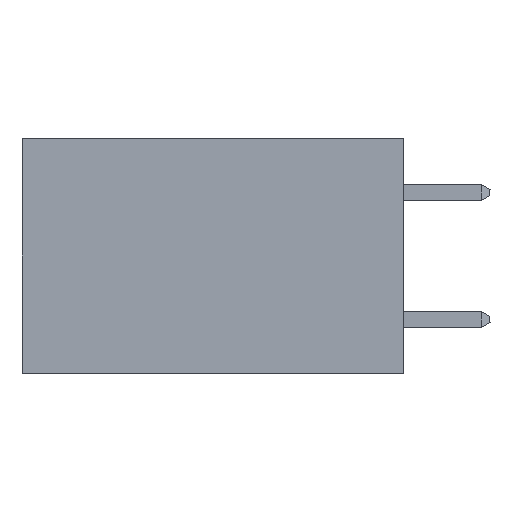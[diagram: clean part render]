
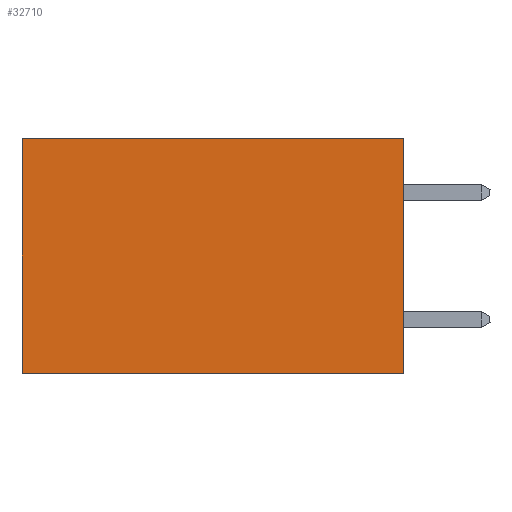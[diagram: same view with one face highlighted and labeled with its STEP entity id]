
A CAD part, left-side view. The second image highlights one B-rep face of the part: STEP entity #32710.
In plain terms, the highlighted planar face has unit normal (-1, 0, 0).
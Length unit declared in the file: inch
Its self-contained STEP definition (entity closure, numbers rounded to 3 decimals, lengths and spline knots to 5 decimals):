
#2787 = ORIENTED_EDGE ( 'NONE', *, *, #8721, .T. ) ;
#2903 = VERTEX_POINT ( 'NONE', #18863 ) ;
#3817 = ORIENTED_EDGE ( 'NONE', *, *, #26472, .T. ) ;
#4316 = CARTESIAN_POINT ( 'NONE',  ( 0.2875, 0.6, -0.37 ) ) ;
#5129 = DIRECTION ( 'NONE',  ( 1., 0., 0. ) ) ;
#7043 = DIRECTION ( 'NONE',  ( 0., 1., 0. ) ) ;
#7102 = CARTESIAN_POINT ( 'NONE',  ( 0.2875, 0., 0. ) ) ;
#7172 = LINE ( 'NONE', #17363, #12682 ) ;
#8721 = EDGE_CURVE ( 'NONE', #2903, #32211, #14900, .T. ) ;
#10259 = DIRECTION ( 'NONE',  ( 0., 0., -1. ) ) ;
#10766 = EDGE_LOOP ( 'NONE', ( #3817, #18517, #32597, #2787 ) ) ;
#11754 = CARTESIAN_POINT ( 'NONE',  ( 0.2875, 0.6, 0. ) ) ;
#12483 = EDGE_CURVE ( 'NONE', #2903, #37569, #7172, .T. ) ;
#12682 = VECTOR ( 'NONE', #14166, 39.37008 ) ;
#14070 = DIRECTION ( 'NONE',  ( 0., 0., -1. ) ) ;
#14166 = DIRECTION ( 'NONE',  ( 0., 0., -1. ) ) ;
#14900 = LINE ( 'NONE', #7102, #30327 ) ;
#16572 = DIRECTION ( 'NONE',  ( 0., 1., 0. ) ) ;
#17088 = VECTOR ( 'NONE', #7043, 39.37008 ) ;
#17363 = CARTESIAN_POINT ( 'NONE',  ( 0.2875, 0., 0. ) ) ;
#18517 = ORIENTED_EDGE ( 'NONE', *, *, #37823, .F. ) ;
#18863 = CARTESIAN_POINT ( 'NONE',  ( 0.2875, 0., 0. ) ) ;
#20298 = VERTEX_POINT ( 'NONE', #4316 ) ;
#20973 = PLANE ( 'NONE',  #25072 ) ;
#24264 = VECTOR ( 'NONE', #10259, 39.37008 ) ;
#24602 = LINE ( 'NONE', #32791, #17088 ) ;
#25072 = AXIS2_PLACEMENT_3D ( 'NONE', #26981, #5129, #14070 ) ;
#26472 = EDGE_CURVE ( 'NONE', #32211, #20298, #32759, .T. ) ;
#26981 = CARTESIAN_POINT ( 'NONE',  ( 0.2875, 0., 0. ) ) ;
#29276 = CARTESIAN_POINT ( 'NONE',  ( 0.2875, 0.6, 0. ) ) ;
#30327 = VECTOR ( 'NONE', #16572, 39.37008 ) ;
#32211 = VERTEX_POINT ( 'NONE', #11754 ) ;
#32597 = ORIENTED_EDGE ( 'NONE', *, *, #12483, .F. ) ;
#32710 = ADVANCED_FACE ( 'NONE', ( #34966 ), #20973, .F. ) ;
#32759 = LINE ( 'NONE', #29276, #24264 ) ;
#32791 = CARTESIAN_POINT ( 'NONE',  ( 0.2875, 0., -0.37 ) ) ;
#34966 = FACE_OUTER_BOUND ( 'NONE', #10766, .T. ) ;
#37095 = CARTESIAN_POINT ( 'NONE',  ( 0.2875, 0., -0.37 ) ) ;
#37569 = VERTEX_POINT ( 'NONE', #37095 ) ;
#37823 = EDGE_CURVE ( 'NONE', #37569, #20298, #24602, .T. ) ;
